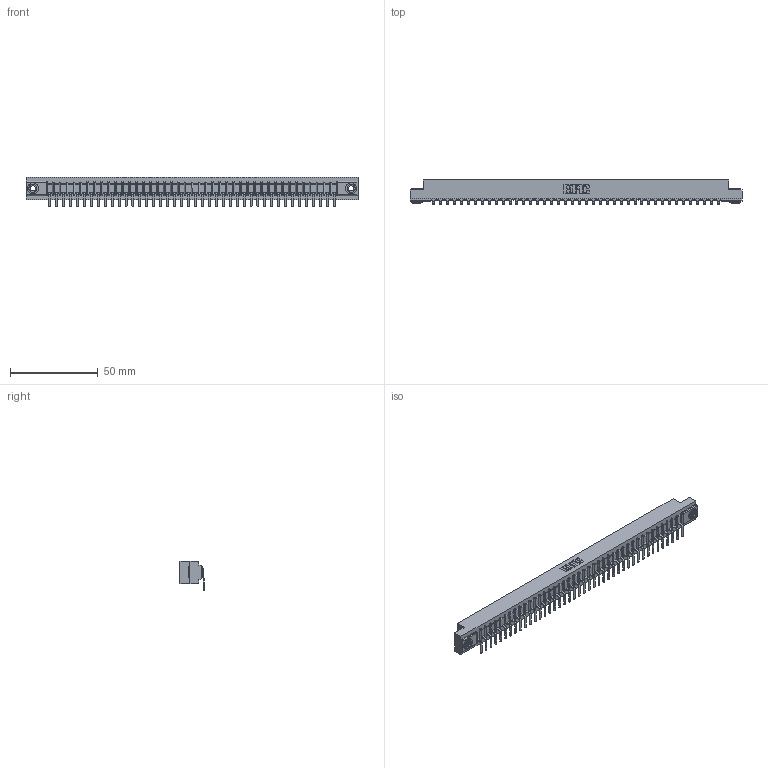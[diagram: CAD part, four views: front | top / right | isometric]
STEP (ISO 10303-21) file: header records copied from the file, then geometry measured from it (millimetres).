
FILE_DESCRIPTION (( 'STEP AP203' ), '1' );
FILE_NAME ('357-042-559-103.STEP', '2022-07-12T19:43:24', ( '' ), ( '' ), 'SwSTEP 2.0', 'SolidWorks 2020', '' );
FILE_SCHEMA (( 'CONFIG_CONTROL_DESIGN' ));
Length unit declared in the file: inch
Products named in the file (4): 345-250-002_345-250-002-102; 357-042-559-103; 307 Part_.156 Dia Mounting Holes; 307-290-001_558 559 - 1 (Single)
Assembly tree (45 placements, depth 2):
  357-042-559-103
    307 Part_.156 Dia Mounting Holes
    307-290-001_558 559 - 1 (Single)  x42
    345-250-002_345-250-002-102  x2
Bounding box: 189.43 x 13.7 x 16.8 mm (x, y, z)
Volume: 19689.7 mm3; surface area: 21214.7 mm2
Topology: 45 solids, 45 shells, 2733 faces, 7743 edges, 4986 vertices
Faces by surface type: plane 1732, cylinder 907, sphere 86, cone 8
Entity records: 37175 total; most frequent: CARTESIAN_POINT 6241, ORIENTED_EDGE 6218, DIRECTION 6085, EDGE_CURVE 3109, VECTOR 2377, LINE 2377, VERTEX_POINT 2010, AXIS2_PLACEMENT_3D 1854
